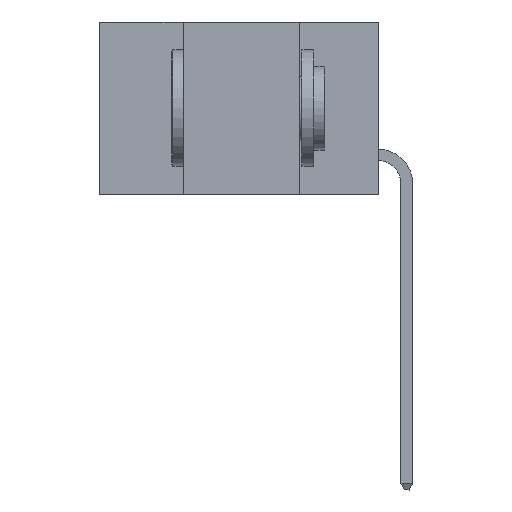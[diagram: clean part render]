
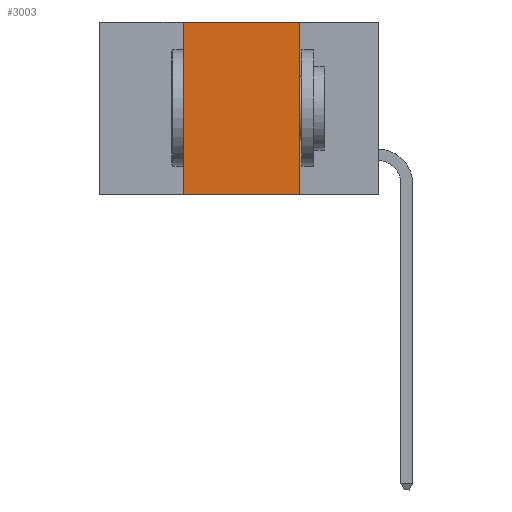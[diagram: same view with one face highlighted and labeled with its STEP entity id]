
A CAD part, left-side view. The second image highlights one B-rep face of the part: STEP entity #3003.
In plain terms, the highlighted planar face has unit normal (-1, 0, 0).
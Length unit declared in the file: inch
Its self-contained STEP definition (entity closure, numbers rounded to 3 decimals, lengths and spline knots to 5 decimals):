
#151 = LINE ( 'NONE', #7589, #2498 ) ;
#206 = VECTOR ( 'NONE', #12188, 39.37008 ) ;
#2231 = VECTOR ( 'NONE', #18950, 39.37008 ) ;
#2498 = VECTOR ( 'NONE', #5175, 39.37008 ) ;
#2808 = CARTESIAN_POINT ( 'NONE',  ( 0., 0.17, -0.37 ) ) ;
#3003 = ADVANCED_FACE ( 'NONE', ( #7874 ), #9945, .F. ) ;
#3501 = EDGE_CURVE ( 'NONE', #22214, #24100, #151, .T. ) ;
#4173 = VECTOR ( 'NONE', #17568, 39.37008 ) ;
#4743 = LINE ( 'NONE', #2808, #206 ) ;
#5175 = DIRECTION ( 'NONE',  ( 0., 0., 1. ) ) ;
#5788 = ORIENTED_EDGE ( 'NONE', *, *, #21464, .F. ) ;
#6287 = DIRECTION ( 'NONE',  ( 1., 0., 0. ) ) ;
#6581 = LINE ( 'NONE', #19654, #4173 ) ;
#7589 = CARTESIAN_POINT ( 'NONE',  ( 0., 0.42, -0.37 ) ) ;
#7874 = FACE_OUTER_BOUND ( 'NONE', #21085, .T. ) ;
#7941 = CARTESIAN_POINT ( 'NONE',  ( 0., 0.6, -0.37 ) ) ;
#9509 = ORIENTED_EDGE ( 'NONE', *, *, #22638, .F. ) ;
#9691 = EDGE_CURVE ( 'NONE', #22214, #12568, #15280, .T. ) ;
#9945 = PLANE ( 'NONE',  #16893 ) ;
#12188 = DIRECTION ( 'NONE',  ( 0., 0., -1. ) ) ;
#12568 = VERTEX_POINT ( 'NONE', #17660 ) ;
#12993 = ORIENTED_EDGE ( 'NONE', *, *, #3501, .F. ) ;
#15280 = LINE ( 'NONE', #7941, #2231 ) ;
#15319 = CARTESIAN_POINT ( 'NONE',  ( 0., 0.6, 0. ) ) ;
#16893 = AXIS2_PLACEMENT_3D ( 'NONE', #15319, #6287, #22809 ) ;
#17282 = CARTESIAN_POINT ( 'NONE',  ( 0., 0.17, 0. ) ) ;
#17378 = CARTESIAN_POINT ( 'NONE',  ( 0., 0.42, -0.37 ) ) ;
#17568 = DIRECTION ( 'NONE',  ( 0., -1., 0. ) ) ;
#17660 = CARTESIAN_POINT ( 'NONE',  ( 0., 0.17, -0.37 ) ) ;
#18950 = DIRECTION ( 'NONE',  ( 0., -1., 0. ) ) ;
#19654 = CARTESIAN_POINT ( 'NONE',  ( 0., 0.6, 0. ) ) ;
#21085 = EDGE_LOOP ( 'NONE', ( #5788, #9509, #12993, #22356 ) ) ;
#21464 = EDGE_CURVE ( 'NONE', #21795, #12568, #4743, .T. ) ;
#21795 = VERTEX_POINT ( 'NONE', #17282 ) ;
#22214 = VERTEX_POINT ( 'NONE', #17378 ) ;
#22338 = CARTESIAN_POINT ( 'NONE',  ( 0., 0.42, 0. ) ) ;
#22356 = ORIENTED_EDGE ( 'NONE', *, *, #9691, .T. ) ;
#22638 = EDGE_CURVE ( 'NONE', #24100, #21795, #6581, .T. ) ;
#22809 = DIRECTION ( 'NONE',  ( 0., 0., -1. ) ) ;
#24100 = VERTEX_POINT ( 'NONE', #22338 ) ;
